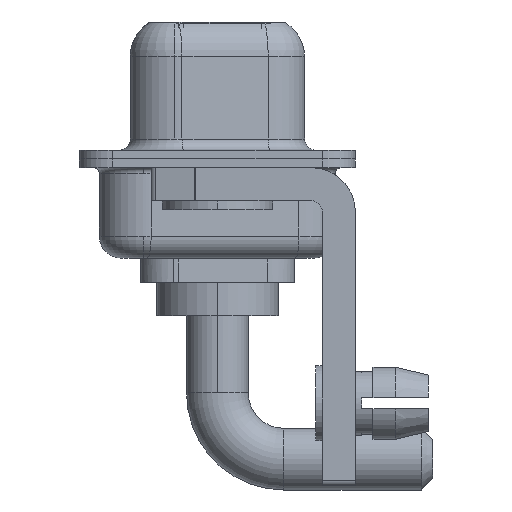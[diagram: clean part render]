
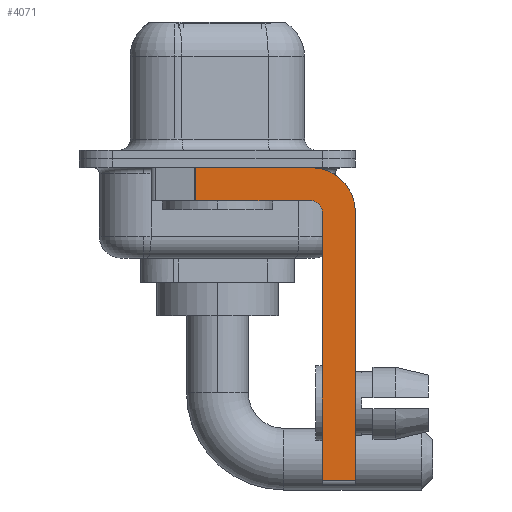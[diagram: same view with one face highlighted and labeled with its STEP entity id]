
A CAD part, left-side view. The second image highlights one B-rep face of the part: STEP entity #4071.
In plain terms, the highlighted planar face has unit normal (-1, 0, 0).
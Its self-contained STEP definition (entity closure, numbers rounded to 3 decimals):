
#177 = DIRECTION ( 'NONE',  ( 0., 0., 1. ) ) ;
#239 = ORIENTED_EDGE ( 'NONE', *, *, #1155, .F. ) ;
#467 = CARTESIAN_POINT ( 'NONE',  ( -2.9, -4.75, -2.4 ) ) ;
#495 = DIRECTION ( 'NONE',  ( 0., 0., -1. ) ) ;
#585 = LINE ( 'NONE', #11376, #4940 ) ;
#614 = VERTEX_POINT ( 'NONE', #12745 ) ;
#1029 = EDGE_CURVE ( 'NONE', #14835, #14479, #1261, .T. ) ;
#1155 = EDGE_CURVE ( 'NONE', #14380, #10748, #8980, .T. ) ;
#1261 = LINE ( 'NONE', #3725, #13991 ) ;
#1391 = FACE_OUTER_BOUND ( 'NONE', #11528, .T. ) ;
#1459 = VERTEX_POINT ( 'NONE', #5695 ) ;
#1544 = CIRCLE ( 'NONE', #9912, 0.5 ) ;
#1654 = CARTESIAN_POINT ( 'NONE',  ( -2.9, -4.25, -2.4 ) ) ;
#1721 = CARTESIAN_POINT ( 'NONE',  ( -2.9, 0.978, -1.9 ) ) ;
#1778 = LINE ( 'NONE', #13834, #11241 ) ;
#2097 = EDGE_CURVE ( 'NONE', #1459, #614, #585, .T. ) ;
#2878 = DIRECTION ( 'NONE',  ( -1., 0., 0. ) ) ;
#3457 = VERTEX_POINT ( 'NONE', #12418 ) ;
#3725 = CARTESIAN_POINT ( 'NONE',  ( -2.9, -4.25, -1.9 ) ) ;
#4014 = DIRECTION ( 'NONE',  ( 0., 0., -1. ) ) ;
#4071 = ADVANCED_FACE ( 'NONE', ( #1391 ), #5119, .F. ) ;
#4170 = AXIS2_PLACEMENT_3D ( 'NONE', #1654, #13784, #11244 ) ;
#4940 = VECTOR ( 'NONE', #5202, 1000. ) ;
#4974 = CARTESIAN_POINT ( 'NONE',  ( -2.9, -6.25, -2.4 ) ) ;
#5119 = PLANE ( 'NONE',  #9556 ) ;
#5202 = DIRECTION ( 'NONE',  ( 0., -1., 0. ) ) ;
#5395 = LINE ( 'NONE', #15053, #12719 ) ;
#5695 = CARTESIAN_POINT ( 'NONE',  ( -2.9, -4.75, -14.55 ) ) ;
#5707 = CARTESIAN_POINT ( 'NONE',  ( -2.9, 3., -0.4 ) ) ;
#6831 = ORIENTED_EDGE ( 'NONE', *, *, #9172, .F. ) ;
#8057 = DIRECTION ( 'NONE',  ( 0., 0., -1. ) ) ;
#8387 = ORIENTED_EDGE ( 'NONE', *, *, #1029, .F. ) ;
#8909 = CARTESIAN_POINT ( 'NONE',  ( -2.9, -4.25, -2.4 ) ) ;
#8939 = LINE ( 'NONE', #1721, #13283 ) ;
#8980 = CIRCLE ( 'NONE', #4170, 2. ) ;
#9045 = DIRECTION ( 'NONE',  ( 0., 0., 1. ) ) ;
#9159 = VERTEX_POINT ( 'NONE', #467 ) ;
#9172 = EDGE_CURVE ( 'NONE', #1459, #9159, #5395, .T. ) ;
#9369 = CARTESIAN_POINT ( 'NONE',  ( -2.9, -4.25, -1.9 ) ) ;
#9556 = AXIS2_PLACEMENT_3D ( 'NONE', #9956, #13601, #4014 ) ;
#9659 = VECTOR ( 'NONE', #15288, 1000. ) ;
#9809 = ORIENTED_EDGE ( 'NONE', *, *, #2097, .T. ) ;
#9912 = AXIS2_PLACEMENT_3D ( 'NONE', #8909, #2878, #177 ) ;
#9956 = CARTESIAN_POINT ( 'NONE',  ( -2.9, -4.25, -2.4 ) ) ;
#10013 = CARTESIAN_POINT ( 'NONE',  ( -2.9, 0.978, -1.9 ) ) ;
#10029 = EDGE_CURVE ( 'NONE', #10748, #614, #1778, .T. ) ;
#10465 = LINE ( 'NONE', #5707, #9659 ) ;
#10748 = VERTEX_POINT ( 'NONE', #4974 ) ;
#10829 = ORIENTED_EDGE ( 'NONE', *, *, #13267, .F. ) ;
#11049 = EDGE_CURVE ( 'NONE', #3457, #14479, #8939, .T. ) ;
#11241 = VECTOR ( 'NONE', #495, 1000. ) ;
#11244 = DIRECTION ( 'NONE',  ( 0., 0., -1. ) ) ;
#11376 = CARTESIAN_POINT ( 'NONE',  ( -2.9, -4.25, -14.55 ) ) ;
#11528 = EDGE_LOOP ( 'NONE', ( #12315, #12616, #8387, #10829, #6831, #9809, #15078, #239 ) ) ;
#12315 = ORIENTED_EDGE ( 'NONE', *, *, #15429, .F. ) ;
#12418 = CARTESIAN_POINT ( 'NONE',  ( -2.9, 0.978, -0.4 ) ) ;
#12616 = ORIENTED_EDGE ( 'NONE', *, *, #11049, .T. ) ;
#12719 = VECTOR ( 'NONE', #9045, 1000. ) ;
#12745 = CARTESIAN_POINT ( 'NONE',  ( -2.9, -6.25, -14.55 ) ) ;
#13221 = DIRECTION ( 'NONE',  ( 0., 1., 0. ) ) ;
#13267 = EDGE_CURVE ( 'NONE', #9159, #14835, #1544, .T. ) ;
#13283 = VECTOR ( 'NONE', #8057, 1000. ) ;
#13601 = DIRECTION ( 'NONE',  ( 1., 0., 0. ) ) ;
#13784 = DIRECTION ( 'NONE',  ( 1., 0., 0. ) ) ;
#13834 = CARTESIAN_POINT ( 'NONE',  ( -2.9, -6.25, -2.4 ) ) ;
#13991 = VECTOR ( 'NONE', #13221, 1000. ) ;
#14380 = VERTEX_POINT ( 'NONE', #14913 ) ;
#14479 = VERTEX_POINT ( 'NONE', #10013 ) ;
#14835 = VERTEX_POINT ( 'NONE', #9369 ) ;
#14913 = CARTESIAN_POINT ( 'NONE',  ( -2.9, -4.25, -0.4 ) ) ;
#15053 = CARTESIAN_POINT ( 'NONE',  ( -2.9, -4.75, -14.8 ) ) ;
#15078 = ORIENTED_EDGE ( 'NONE', *, *, #10029, .F. ) ;
#15288 = DIRECTION ( 'NONE',  ( 0., -1., 0. ) ) ;
#15429 = EDGE_CURVE ( 'NONE', #3457, #14380, #10465, .T. ) ;
